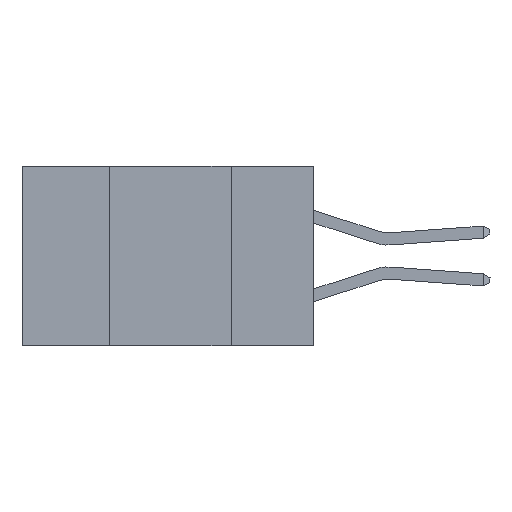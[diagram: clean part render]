
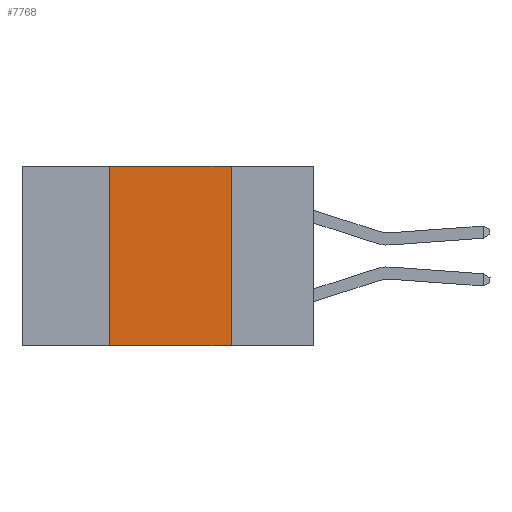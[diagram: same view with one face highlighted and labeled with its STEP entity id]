
A CAD part, left-side view. The second image highlights one B-rep face of the part: STEP entity #7768.
In plain terms, the highlighted planar face has unit normal (-1, 0, 0).
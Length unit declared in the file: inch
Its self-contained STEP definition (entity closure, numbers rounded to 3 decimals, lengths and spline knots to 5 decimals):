
#458 = VERTEX_POINT ( 'NONE', #5648 ) ;
#565 = EDGE_CURVE ( 'NONE', #458, #4559, #5391, .T. ) ;
#1541 = AXIS2_PLACEMENT_3D ( 'NONE', #3212, #9329, #1869 ) ;
#1727 = EDGE_CURVE ( 'NONE', #12227, #4559, #11433, .T. ) ;
#1869 = DIRECTION ( 'NONE',  ( 0., 0., -1. ) ) ;
#2299 = CARTESIAN_POINT ( 'NONE',  ( 0., 0.17, 0. ) ) ;
#3140 = ORIENTED_EDGE ( 'NONE', *, *, #565, .T. ) ;
#3212 = CARTESIAN_POINT ( 'NONE',  ( 0., 0.6, 0. ) ) ;
#3583 = CARTESIAN_POINT ( 'NONE',  ( 0., 0.17, 0. ) ) ;
#3809 = ORIENTED_EDGE ( 'NONE', *, *, #19238, .F. ) ;
#4559 = VERTEX_POINT ( 'NONE', #8541 ) ;
#4921 = ORIENTED_EDGE ( 'NONE', *, *, #7019, .F. ) ;
#5391 = LINE ( 'NONE', #11194, #6310 ) ;
#5648 = CARTESIAN_POINT ( 'NONE',  ( 0., 0.42, -0.37 ) ) ;
#5825 = VECTOR ( 'NONE', #6532, 39.37008 ) ;
#6310 = VECTOR ( 'NONE', #8248, 39.37008 ) ;
#6532 = DIRECTION ( 'NONE',  ( 0., -1., 0. ) ) ;
#7019 = EDGE_CURVE ( 'NONE', #9315, #12227, #17868, .T. ) ;
#7069 = EDGE_LOOP ( 'NONE', ( #17046, #4921, #3809, #3140 ) ) ;
#7427 = FACE_OUTER_BOUND ( 'NONE', #7069, .T. ) ;
#7436 = VECTOR ( 'NONE', #17006, 39.37008 ) ;
#7768 = ADVANCED_FACE ( 'NONE', ( #7427 ), #7780, .F. ) ;
#7780 = PLANE ( 'NONE',  #1541 ) ;
#7945 = CARTESIAN_POINT ( 'NONE',  ( 0., 0.6, 0. ) ) ;
#8248 = DIRECTION ( 'NONE',  ( 0., -1., 0. ) ) ;
#8289 = CARTESIAN_POINT ( 'NONE',  ( 0., 0.42, 0. ) ) ;
#8541 = CARTESIAN_POINT ( 'NONE',  ( 0., 0.17, -0.37 ) ) ;
#9315 = VERTEX_POINT ( 'NONE', #8289 ) ;
#9329 = DIRECTION ( 'NONE',  ( 1., 0., 0. ) ) ;
#10258 = VECTOR ( 'NONE', #14873, 39.37008 ) ;
#11194 = CARTESIAN_POINT ( 'NONE',  ( 0., 0.6, -0.37 ) ) ;
#11433 = LINE ( 'NONE', #3583, #7436 ) ;
#12227 = VERTEX_POINT ( 'NONE', #2299 ) ;
#14311 = LINE ( 'NONE', #14806, #10258 ) ;
#14806 = CARTESIAN_POINT ( 'NONE',  ( 0., 0.42, 0. ) ) ;
#14873 = DIRECTION ( 'NONE',  ( 0., 0., 1. ) ) ;
#17006 = DIRECTION ( 'NONE',  ( 0., 0., -1. ) ) ;
#17046 = ORIENTED_EDGE ( 'NONE', *, *, #1727, .F. ) ;
#17868 = LINE ( 'NONE', #7945, #5825 ) ;
#19238 = EDGE_CURVE ( 'NONE', #458, #9315, #14311, .T. ) ;
